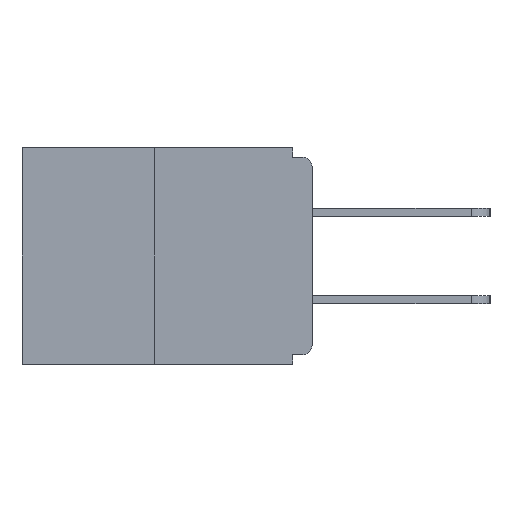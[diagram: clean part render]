
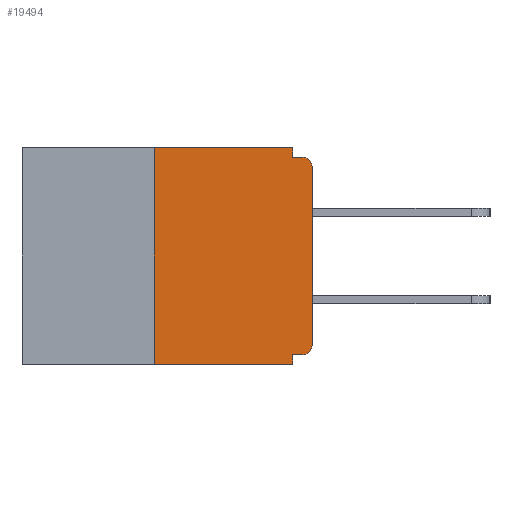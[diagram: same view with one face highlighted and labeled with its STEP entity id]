
A CAD part, left-side view. The second image highlights one B-rep face of the part: STEP entity #19494.
In plain terms, the highlighted planar face has unit normal (-1, 0, 0).
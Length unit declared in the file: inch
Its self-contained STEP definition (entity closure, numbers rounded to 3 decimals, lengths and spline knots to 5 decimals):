
#688 = ORIENTED_EDGE ( 'NONE', *, *, #22416, .F. ) ;
#1190 = VECTOR ( 'NONE', #10734, 39.37008 ) ;
#1327 = LINE ( 'NONE', #25772, #15581 ) ;
#1336 = EDGE_CURVE ( 'NONE', #22319, #6000, #26689, .T. ) ;
#1971 = ORIENTED_EDGE ( 'NONE', *, *, #24748, .T. ) ;
#2164 = CARTESIAN_POINT ( 'NONE',  ( 0., 0., -0.015 ) ) ;
#2207 = CARTESIAN_POINT ( 'NONE',  ( 0., 0.25, -0.343 ) ) ;
#3267 = ORIENTED_EDGE ( 'NONE', *, *, #17011, .T. ) ;
#3720 = DIRECTION ( 'NONE',  ( -1., 0., 0. ) ) ;
#4028 = CARTESIAN_POINT ( 'NONE',  ( 0., 0., 0. ) ) ;
#4258 = LINE ( 'NONE', #2164, #16176 ) ;
#4487 = ORIENTED_EDGE ( 'NONE', *, *, #25498, .F. ) ;
#4621 = DIRECTION ( 'NONE',  ( 1., 0., 0. ) ) ;
#5975 = EDGE_CURVE ( 'NONE', #18513, #9468, #15559, .T. ) ;
#6000 = VERTEX_POINT ( 'NONE', #6473 ) ;
#6432 = CARTESIAN_POINT ( 'NONE',  ( 0., 0.031, 0. ) ) ;
#6473 = CARTESIAN_POINT ( 'NONE',  ( 0., 0.031, -0.343 ) ) ;
#6752 = EDGE_CURVE ( 'NONE', #20394, #17111, #25157, .T. ) ;
#7000 = VERTEX_POINT ( 'NONE', #6432 ) ;
#7019 = EDGE_CURVE ( 'NONE', #26145, #17111, #4258, .T. ) ;
#7623 = CARTESIAN_POINT ( 'NONE',  ( 0., 0.015, -0.03 ) ) ;
#7659 = EDGE_CURVE ( 'NONE', #22319, #20663, #27104, .T. ) ;
#7712 = DIRECTION ( 'NONE',  ( 0., 0., -1. ) ) ;
#7835 = ORIENTED_EDGE ( 'NONE', *, *, #6752, .T. ) ;
#9468 = VERTEX_POINT ( 'NONE', #18517 ) ;
#9655 = AXIS2_PLACEMENT_3D ( 'NONE', #27025, #3720, #17630 ) ;
#9748 = VECTOR ( 'NONE', #19045, 39.37008 ) ;
#9897 = CARTESIAN_POINT ( 'NONE',  ( 0., 0.031, -0.343 ) ) ;
#10049 = VERTEX_POINT ( 'NONE', #17923 ) ;
#10263 = DIRECTION ( 'NONE',  ( 0., 0., -1. ) ) ;
#10410 = ORIENTED_EDGE ( 'NONE', *, *, #5975, .F. ) ;
#10734 = DIRECTION ( 'NONE',  ( 0., 0., 1. ) ) ;
#11786 = CARTESIAN_POINT ( 'NONE',  ( 0., 0.46, 0. ) ) ;
#11808 = EDGE_CURVE ( 'NONE', #7000, #26145, #27043, .T. ) ;
#11874 = EDGE_LOOP ( 'NONE', ( #688, #19824, #22109, #4487, #10410, #3267, #1971, #7835, #26462, #22102 ) ) ;
#12285 = CIRCLE ( 'NONE', #9655, 0.015 ) ;
#12336 = DIRECTION ( 'NONE',  ( 0., -1., 0. ) ) ;
#12706 = DIRECTION ( 'NONE',  ( 0., 1., 0. ) ) ;
#12798 = FACE_OUTER_BOUND ( 'NONE', #11874, .T. ) ;
#13048 = AXIS2_PLACEMENT_3D ( 'NONE', #7623, #27038, #7712 ) ;
#13054 = AXIS2_PLACEMENT_3D ( 'NONE', #11786, #4621, #10263 ) ;
#14364 = DIRECTION ( 'NONE',  ( 0., 0., -1. ) ) ;
#14474 = DIRECTION ( 'NONE',  ( 0., 0., 1. ) ) ;
#14837 = VECTOR ( 'NONE', #14474, 39.37008 ) ;
#15535 = LINE ( 'NONE', #9897, #18165 ) ;
#15559 = LINE ( 'NONE', #19192, #26550 ) ;
#15581 = VECTOR ( 'NONE', #21723, 39.37008 ) ;
#15857 = CARTESIAN_POINT ( 'NONE',  ( 0., 0., -0.03 ) ) ;
#16176 = VECTOR ( 'NONE', #17027, 39.37008 ) ;
#16643 = CARTESIAN_POINT ( 'NONE',  ( 0., 0.031, -0.015 ) ) ;
#16826 = CARTESIAN_POINT ( 'NONE',  ( 0., 0.031, 0. ) ) ;
#17011 = EDGE_CURVE ( 'NONE', #18513, #10049, #12285, .T. ) ;
#17027 = DIRECTION ( 'NONE',  ( 0., -1., 0. ) ) ;
#17111 = VERTEX_POINT ( 'NONE', #26989 ) ;
#17630 = DIRECTION ( 'NONE',  ( 0., 0., -1. ) ) ;
#17923 = CARTESIAN_POINT ( 'NONE',  ( 0., 0., -0.313 ) ) ;
#18165 = VECTOR ( 'NONE', #14364, 39.37008 ) ;
#18513 = VERTEX_POINT ( 'NONE', #23116 ) ;
#18517 = CARTESIAN_POINT ( 'NONE',  ( 0., 0.031, -0.328 ) ) ;
#19045 = DIRECTION ( 'NONE',  ( 0., 0., -1. ) ) ;
#19192 = CARTESIAN_POINT ( 'NONE',  ( 0., 0., -0.328 ) ) ;
#19494 = ADVANCED_FACE ( 'NONE', ( #12798 ), #26823, .F. ) ;
#19696 = VECTOR ( 'NONE', #12336, 39.37008 ) ;
#19824 = ORIENTED_EDGE ( 'NONE', *, *, #7659, .F. ) ;
#20394 = VERTEX_POINT ( 'NONE', #15857 ) ;
#20663 = VERTEX_POINT ( 'NONE', #25907 ) ;
#21723 = DIRECTION ( 'NONE',  ( 0., -1., 0. ) ) ;
#22102 = ORIENTED_EDGE ( 'NONE', *, *, #11808, .F. ) ;
#22109 = ORIENTED_EDGE ( 'NONE', *, *, #1336, .T. ) ;
#22319 = VERTEX_POINT ( 'NONE', #2207 ) ;
#22416 = EDGE_CURVE ( 'NONE', #20663, #7000, #1327, .T. ) ;
#22460 = CARTESIAN_POINT ( 'NONE',  ( 0., 0.25, 0. ) ) ;
#22873 = CARTESIAN_POINT ( 'NONE',  ( 0., 0.46, -0.343 ) ) ;
#23116 = CARTESIAN_POINT ( 'NONE',  ( 0., 0.015, -0.328 ) ) ;
#24748 = EDGE_CURVE ( 'NONE', #10049, #20394, #27440, .T. ) ;
#25157 = CIRCLE ( 'NONE', #13048, 0.015 ) ;
#25498 = EDGE_CURVE ( 'NONE', #9468, #6000, #15535, .T. ) ;
#25772 = CARTESIAN_POINT ( 'NONE',  ( 0., 0.46, 0. ) ) ;
#25907 = CARTESIAN_POINT ( 'NONE',  ( 0., 0.25, 0. ) ) ;
#26145 = VERTEX_POINT ( 'NONE', #16643 ) ;
#26462 = ORIENTED_EDGE ( 'NONE', *, *, #7019, .F. ) ;
#26550 = VECTOR ( 'NONE', #12706, 39.37008 ) ;
#26689 = LINE ( 'NONE', #22873, #19696 ) ;
#26823 = PLANE ( 'NONE',  #13054 ) ;
#26989 = CARTESIAN_POINT ( 'NONE',  ( 0., 0.015, -0.015 ) ) ;
#27025 = CARTESIAN_POINT ( 'NONE',  ( 0., 0.015, -0.313 ) ) ;
#27038 = DIRECTION ( 'NONE',  ( -1., 0., 0. ) ) ;
#27043 = LINE ( 'NONE', #16826, #9748 ) ;
#27104 = LINE ( 'NONE', #22460, #14837 ) ;
#27440 = LINE ( 'NONE', #4028, #1190 ) ;
